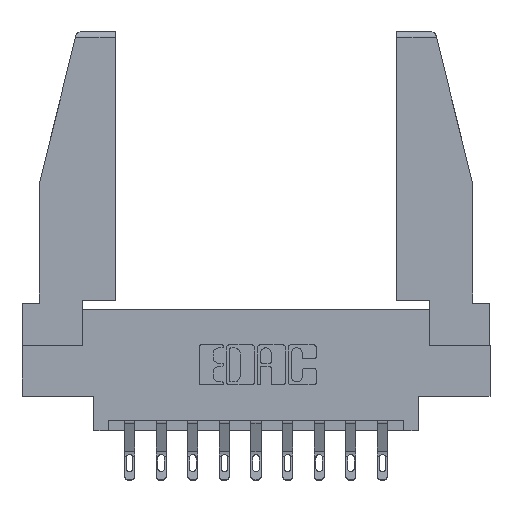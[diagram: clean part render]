
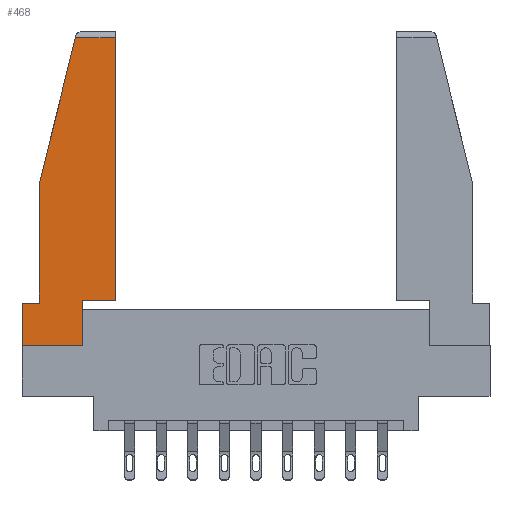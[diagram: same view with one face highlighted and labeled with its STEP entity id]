
A CAD part, top view. The second image highlights one B-rep face of the part: STEP entity #468.
In plain terms, the highlighted planar face has unit normal (0, 0, 1).
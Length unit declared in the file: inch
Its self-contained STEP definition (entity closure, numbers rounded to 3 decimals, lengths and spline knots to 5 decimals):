
#134 = DIRECTION ( 'NONE',  ( 1., 0., 0. ) ) ;
#190 = EDGE_CURVE ( 'NONE', #3802, #4904, #9998, .T. ) ;
#326 = ORIENTED_EDGE ( 'NONE', *, *, #13971, .T. ) ;
#377 = VECTOR ( 'NONE', #6963, 39.37008 ) ;
#410 = VERTEX_POINT ( 'NONE', #5505 ) ;
#468 = ADVANCED_FACE ( 'NONE', ( #8599 ), #13635, .T. ) ;
#589 = DIRECTION ( 'NONE',  ( 0., 0., 1. ) ) ;
#606 = EDGE_CURVE ( 'NONE', #7793, #5995, #9468, .T. ) ;
#1019 = VERTEX_POINT ( 'NONE', #12729 ) ;
#1184 = LINE ( 'NONE', #6480, #2341 ) ;
#1238 = LINE ( 'NONE', #12442, #6698 ) ;
#1592 = VERTEX_POINT ( 'NONE', #9411 ) ;
#1684 = CARTESIAN_POINT ( 'NONE',  ( 0., 0., 0. ) ) ;
#1825 = CARTESIAN_POINT ( 'NONE',  ( 0.297, 0., 0. ) ) ;
#2101 = LINE ( 'NONE', #13686, #3408 ) ;
#2250 = LINE ( 'NONE', #2481, #6705 ) ;
#2341 = VECTOR ( 'NONE', #5546, 39.37008 ) ;
#2481 = CARTESIAN_POINT ( 'NONE',  ( 0.086, 0.8, 0. ) ) ;
#2839 = EDGE_CURVE ( 'NONE', #4904, #7793, #7417, .T. ) ;
#2886 = EDGE_CURVE ( 'NONE', #5995, #1019, #10702, .T. ) ;
#3231 = DIRECTION ( 'NONE',  ( 1., 0., 0. ) ) ;
#3334 = CARTESIAN_POINT ( 'NONE',  ( 0., 0., 0. ) ) ;
#3408 = VECTOR ( 'NONE', #9316, 39.37008 ) ;
#3802 = VERTEX_POINT ( 'NONE', #8469 ) ;
#3948 = AXIS2_PLACEMENT_3D ( 'NONE', #10410, #589, #4909 ) ;
#4321 = CARTESIAN_POINT ( 'NONE',  ( 0.297, 0., 0. ) ) ;
#4562 = EDGE_CURVE ( 'NONE', #1592, #12866, #2250, .T. ) ;
#4789 = CARTESIAN_POINT ( 'NONE',  ( 0., 0.21, 0. ) ) ;
#4828 = VERTEX_POINT ( 'NONE', #13674 ) ;
#4904 = VERTEX_POINT ( 'NONE', #1684 ) ;
#4909 = DIRECTION ( 'NONE',  ( 1., 0., 0. ) ) ;
#4976 = VECTOR ( 'NONE', #13483, 39.37008 ) ;
#5088 = DIRECTION ( 'NONE',  ( 0., -1., 0. ) ) ;
#5149 = LINE ( 'NONE', #4789, #4976 ) ;
#5505 = CARTESIAN_POINT ( 'NONE',  ( 0.461, 1.52, 0. ) ) ;
#5546 = DIRECTION ( 'NONE',  ( -1., 0., 0. ) ) ;
#5550 = EDGE_CURVE ( 'NONE', #1019, #410, #2101, .T. ) ;
#5867 = VECTOR ( 'NONE', #5088, 39.37008 ) ;
#5930 = CARTESIAN_POINT ( 'NONE',  ( 0.086, 0.21, 0. ) ) ;
#5995 = VERTEX_POINT ( 'NONE', #13469 ) ;
#6286 = ORIENTED_EDGE ( 'NONE', *, *, #13857, .T. ) ;
#6480 = CARTESIAN_POINT ( 'NONE',  ( 0., 1.52, 0. ) ) ;
#6696 = CARTESIAN_POINT ( 'NONE',  ( 0.297, 0.223, 0. ) ) ;
#6698 = VECTOR ( 'NONE', #9415, 39.37008 ) ;
#6705 = VECTOR ( 'NONE', #13644, 39.37008 ) ;
#6963 = DIRECTION ( 'NONE',  ( 0., 1., 0. ) ) ;
#7417 = LINE ( 'NONE', #3334, #11737 ) ;
#7532 = ORIENTED_EDGE ( 'NONE', *, *, #2839, .T. ) ;
#7742 = VECTOR ( 'NONE', #134, 39.37008 ) ;
#7793 = VERTEX_POINT ( 'NONE', #1825 ) ;
#8135 = ORIENTED_EDGE ( 'NONE', *, *, #2886, .T. ) ;
#8469 = CARTESIAN_POINT ( 'NONE',  ( 0., 0.21, 0. ) ) ;
#8599 = FACE_OUTER_BOUND ( 'NONE', #12782, .T. ) ;
#9316 = DIRECTION ( 'NONE',  ( 0., 1., 0. ) ) ;
#9411 = CARTESIAN_POINT ( 'NONE',  ( 0.086, 0.8, 0. ) ) ;
#9415 = DIRECTION ( 'NONE',  ( -0.239, -0.971, 0. ) ) ;
#9468 = LINE ( 'NONE', #4321, #377 ) ;
#9745 = ORIENTED_EDGE ( 'NONE', *, *, #606, .T. ) ;
#9998 = LINE ( 'NONE', #10689, #5867 ) ;
#10179 = EDGE_CURVE ( 'NONE', #410, #4828, #1184, .T. ) ;
#10410 = CARTESIAN_POINT ( 'NONE',  ( 0., 0., 0. ) ) ;
#10689 = CARTESIAN_POINT ( 'NONE',  ( 0., 0.21, 0. ) ) ;
#10702 = LINE ( 'NONE', #6696, #7742 ) ;
#10905 = ORIENTED_EDGE ( 'NONE', *, *, #10179, .T. ) ;
#11737 = VECTOR ( 'NONE', #3231, 39.37008 ) ;
#12442 = CARTESIAN_POINT ( 'NONE',  ( 0.271, 1.55, 0. ) ) ;
#12729 = CARTESIAN_POINT ( 'NONE',  ( 0.461, 0.223, 0. ) ) ;
#12782 = EDGE_LOOP ( 'NONE', ( #13659, #10905, #326, #13186, #6286, #12906, #7532, #9745, #8135 ) ) ;
#12866 = VERTEX_POINT ( 'NONE', #5930 ) ;
#12906 = ORIENTED_EDGE ( 'NONE', *, *, #190, .T. ) ;
#13186 = ORIENTED_EDGE ( 'NONE', *, *, #4562, .T. ) ;
#13469 = CARTESIAN_POINT ( 'NONE',  ( 0.297, 0.223, 0. ) ) ;
#13483 = DIRECTION ( 'NONE',  ( -1., 0., 0. ) ) ;
#13635 = PLANE ( 'NONE',  #3948 ) ;
#13644 = DIRECTION ( 'NONE',  ( 0., -1., 0. ) ) ;
#13659 = ORIENTED_EDGE ( 'NONE', *, *, #5550, .T. ) ;
#13674 = CARTESIAN_POINT ( 'NONE',  ( 0.2636, 1.52, 0. ) ) ;
#13686 = CARTESIAN_POINT ( 'NONE',  ( 0.461, 0.223, 0. ) ) ;
#13857 = EDGE_CURVE ( 'NONE', #12866, #3802, #5149, .T. ) ;
#13971 = EDGE_CURVE ( 'NONE', #4828, #1592, #1238, .T. ) ;
